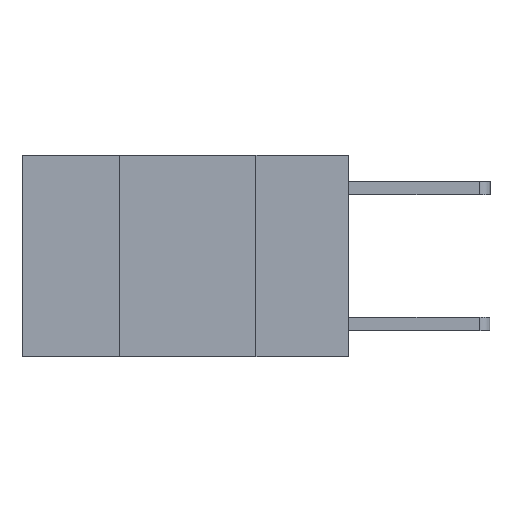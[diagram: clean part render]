
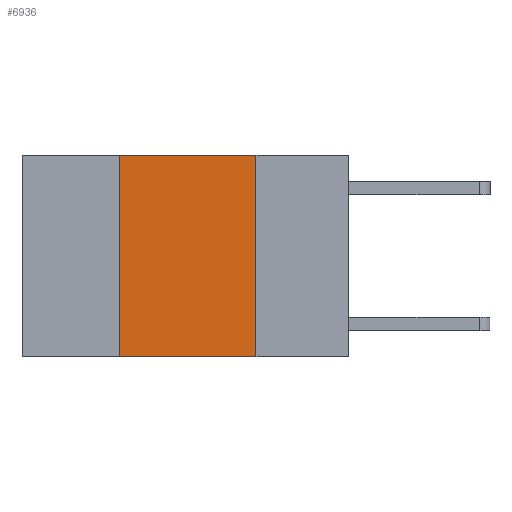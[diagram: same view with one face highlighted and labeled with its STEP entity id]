
A CAD part, left-side view. The second image highlights one B-rep face of the part: STEP entity #6936.
In plain terms, the highlighted planar face has unit normal (-1, 0, 0).
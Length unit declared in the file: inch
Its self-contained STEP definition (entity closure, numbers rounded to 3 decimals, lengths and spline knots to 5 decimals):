
#459 = VECTOR ( 'NONE', #3039, 39.37008 ) ;
#464 = LINE ( 'NONE', #925, #459 ) ;
#791 = VECTOR ( 'NONE', #1269, 39.37008 ) ;
#914 = LINE ( 'NONE', #1282, #791 ) ;
#925 = CARTESIAN_POINT ( 'NONE',  ( 0., 0.42, 0. ) ) ;
#1184 = FACE_OUTER_BOUND ( 'NONE', #6982, .T. ) ;
#1269 = DIRECTION ( 'NONE',  ( 0., 0., -1. ) ) ;
#1282 = CARTESIAN_POINT ( 'NONE',  ( 0., 0.17, 0. ) ) ;
#1336 = CARTESIAN_POINT ( 'NONE',  ( 0., 0.6, -0.37 ) ) ;
#1369 = EDGE_CURVE ( 'NONE', #5211, #3183, #464, .T. ) ;
#1549 = DIRECTION ( 'NONE',  ( 0., -1., 0. ) ) ;
#1642 = EDGE_CURVE ( 'NONE', #5211, #5777, #6598, .T. ) ;
#1691 = VECTOR ( 'NONE', #8110, 39.37008 ) ;
#1886 = LINE ( 'NONE', #5656, #1691 ) ;
#1996 = DIRECTION ( 'NONE',  ( 0., 0., -1. ) ) ;
#2020 = DIRECTION ( 'NONE',  ( 1., 0., 0. ) ) ;
#2134 = PLANE ( 'NONE',  #6618 ) ;
#2248 = CARTESIAN_POINT ( 'NONE',  ( 0., 0.42, 0. ) ) ;
#2249 = CARTESIAN_POINT ( 'NONE',  ( 0., 0.6, 0. ) ) ;
#2464 = EDGE_CURVE ( 'NONE', #3183, #5270, #1886, .T. ) ;
#3039 = DIRECTION ( 'NONE',  ( 0., 0., 1. ) ) ;
#3183 = VERTEX_POINT ( 'NONE', #2248 ) ;
#5211 = VERTEX_POINT ( 'NONE', #8191 ) ;
#5270 = VERTEX_POINT ( 'NONE', #7323 ) ;
#5610 = ORIENTED_EDGE ( 'NONE', *, *, #7036, .F. ) ;
#5656 = CARTESIAN_POINT ( 'NONE',  ( 0., 0.6, 0. ) ) ;
#5777 = VERTEX_POINT ( 'NONE', #6960 ) ;
#5902 = ORIENTED_EDGE ( 'NONE', *, *, #2464, .F. ) ;
#6253 = VECTOR ( 'NONE', #1549, 39.37008 ) ;
#6444 = ORIENTED_EDGE ( 'NONE', *, *, #1642, .T. ) ;
#6598 = LINE ( 'NONE', #1336, #6253 ) ;
#6607 = ORIENTED_EDGE ( 'NONE', *, *, #1369, .F. ) ;
#6618 = AXIS2_PLACEMENT_3D ( 'NONE', #2249, #2020, #1996 ) ;
#6936 = ADVANCED_FACE ( 'NONE', ( #1184 ), #2134, .F. ) ;
#6960 = CARTESIAN_POINT ( 'NONE',  ( 0., 0.17, -0.37 ) ) ;
#6982 = EDGE_LOOP ( 'NONE', ( #5610, #5902, #6607, #6444 ) ) ;
#7036 = EDGE_CURVE ( 'NONE', #5270, #5777, #914, .T. ) ;
#7323 = CARTESIAN_POINT ( 'NONE',  ( 0., 0.17, 0. ) ) ;
#8110 = DIRECTION ( 'NONE',  ( 0., -1., 0. ) ) ;
#8191 = CARTESIAN_POINT ( 'NONE',  ( 0., 0.42, -0.37 ) ) ;
